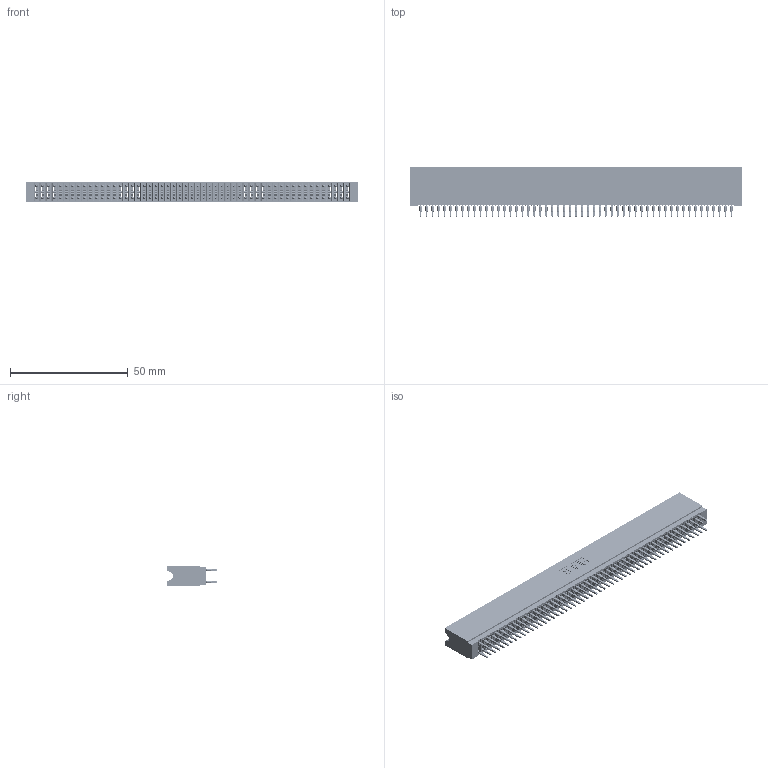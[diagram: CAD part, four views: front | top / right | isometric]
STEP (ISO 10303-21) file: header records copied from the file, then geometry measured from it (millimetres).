
FILE_DESCRIPTION (( 'STEP AP203' ), '1' );
FILE_NAME ('745-106-560-206.STEP', '2026-02-27T00:01:55', ( '' ), ( '' ), 'SwSTEP 2.0', 'SolidWorks 2023', '' );
FILE_SCHEMA (( 'CONFIG_CONTROL_DESIGN' ));
Length unit declared in the file: millimetre
Products named in the file (3): 745-292-001_560; 745-106-560-206; 745 Part_Insulator Option - 06
Assembly tree (107 placements, depth 2):
  745-106-560-206
    745 Part_Insulator Option - 06
    745-292-001_560  x106
Bounding box: 141.22 x 21.22 x 8.89 mm (x, y, z)
Volume: 13021.3 mm3; surface area: 28425.3 mm2
Topology: 107 solids, 107 shells, 10537 faces, 28827 edges, 18298 vertices
Faces by surface type: plane 5462, cylinder 2319, bspline 2120, torus 636
Entity records: 88068 total; most frequent: CARTESIAN_POINT 15776, ORIENTED_EDGE 15234, DIRECTION 13303, EDGE_CURVE 7617, VECTOR 7109, LINE 7109, VERTEX_POINT 4858, AXIS2_PLACEMENT_3D 3097
